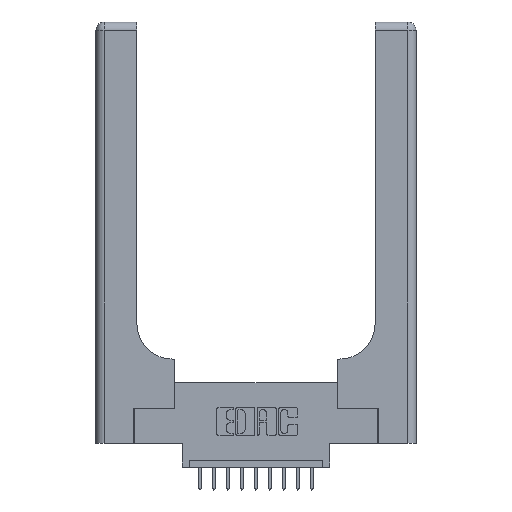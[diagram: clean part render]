
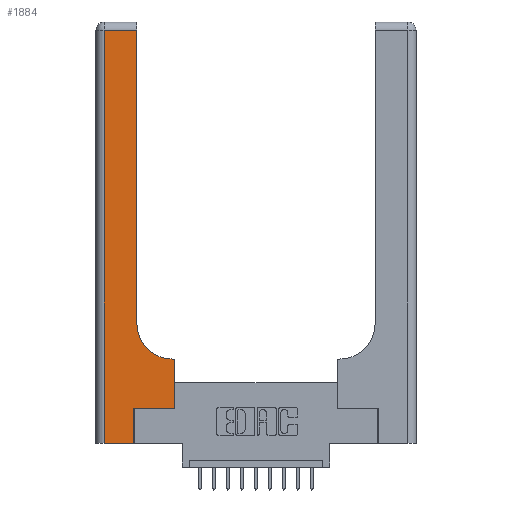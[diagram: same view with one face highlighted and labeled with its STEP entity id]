
A CAD part, top view. The second image highlights one B-rep face of the part: STEP entity #1884.
In plain terms, the highlighted planar face has unit normal (0, 0, 1).
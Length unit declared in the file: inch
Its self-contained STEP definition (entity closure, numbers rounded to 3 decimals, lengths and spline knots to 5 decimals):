
#224 = CARTESIAN_POINT ( 'NONE',  ( 0.2915, 0.6, 0.37 ) ) ;
#412 = VECTOR ( 'NONE', #5298, 39.37008 ) ;
#674 = FACE_OUTER_BOUND ( 'NONE', #16496, .T. ) ;
#1247 = EDGE_CURVE ( 'NONE', #13207, #6034, #7113, .T. ) ;
#1469 = VERTEX_POINT ( 'NONE', #1929 ) ;
#1557 = CARTESIAN_POINT ( 'NONE',  ( 0.06, 0., 0.37 ) ) ;
#1884 = ADVANCED_FACE ( 'NONE', ( #674 ), #8360, .F. ) ;
#1929 = CARTESIAN_POINT ( 'NONE',  ( 0.06, 2.94, 0.37 ) ) ;
#2017 = DIRECTION ( 'NONE',  ( -1., 0., 0. ) ) ;
#2790 = CARTESIAN_POINT ( 'NONE',  ( 0.2915, 3., 0.37 ) ) ;
#2985 = CARTESIAN_POINT ( 'NONE',  ( 0.5585, 0.25, 0.37 ) ) ;
#3104 = DIRECTION ( 'NONE',  ( 0., 1., 0. ) ) ;
#3157 = VECTOR ( 'NONE', #4562, 39.37008 ) ;
#3801 = EDGE_CURVE ( 'NONE', #5965, #1469, #4281, .T. ) ;
#3925 = CARTESIAN_POINT ( 'NONE',  ( 0.5415, 0.6, 0.37 ) ) ;
#3981 = DIRECTION ( 'NONE',  ( -1., 0., 0. ) ) ;
#4088 = DIRECTION ( 'NONE',  ( 0., 1., 0. ) ) ;
#4189 = CARTESIAN_POINT ( 'NONE',  ( 0.5415, 0.85, 0.37 ) ) ;
#4281 = LINE ( 'NONE', #15075, #5456 ) ;
#4562 = DIRECTION ( 'NONE',  ( 0., 1., 0. ) ) ;
#4927 = ORIENTED_EDGE ( 'NONE', *, *, #10710, .T. ) ;
#5298 = DIRECTION ( 'NONE',  ( 1., 0., 0. ) ) ;
#5456 = VECTOR ( 'NONE', #7388, 39.37008 ) ;
#5472 = LINE ( 'NONE', #10953, #6262 ) ;
#5574 = VERTEX_POINT ( 'NONE', #3925 ) ;
#5611 = ORIENTED_EDGE ( 'NONE', *, *, #8566, .T. ) ;
#5673 = LINE ( 'NONE', #2790, #9838 ) ;
#5813 = DIRECTION ( 'NONE',  ( 0., 0., -1. ) ) ;
#5936 = DIRECTION ( 'NONE',  ( 0., -1., 0. ) ) ;
#5965 = VERTEX_POINT ( 'NONE', #11740 ) ;
#5984 = CARTESIAN_POINT ( 'NONE',  ( 0.269, 0., 0.37 ) ) ;
#6010 = CARTESIAN_POINT ( 'NONE',  ( 0.269, 0.25, 0.37 ) ) ;
#6034 = VERTEX_POINT ( 'NONE', #6010 ) ;
#6070 = LINE ( 'NONE', #2985, #13276 ) ;
#6248 = ORIENTED_EDGE ( 'NONE', *, *, #9788, .T. ) ;
#6262 = VECTOR ( 'NONE', #5936, 39.37008 ) ;
#6464 = VECTOR ( 'NONE', #3981, 39.37008 ) ;
#7108 = ORIENTED_EDGE ( 'NONE', *, *, #3801, .T. ) ;
#7113 = LINE ( 'NONE', #5984, #3157 ) ;
#7388 = DIRECTION ( 'NONE',  ( -1., 0., 0. ) ) ;
#8030 = LINE ( 'NONE', #14194, #412 ) ;
#8059 = ORIENTED_EDGE ( 'NONE', *, *, #14907, .T. ) ;
#8360 = PLANE ( 'NONE',  #12251 ) ;
#8391 = CARTESIAN_POINT ( 'NONE',  ( 0.5585, 0.25, 0.37 ) ) ;
#8566 = EDGE_CURVE ( 'NONE', #5574, #14475, #8682, .T. ) ;
#8589 = VERTEX_POINT ( 'NONE', #15667 ) ;
#8682 = CIRCLE ( 'NONE', #15657, 0.25 ) ;
#9118 = ORIENTED_EDGE ( 'NONE', *, *, #1247, .T. ) ;
#9221 = LINE ( 'NONE', #224, #6464 ) ;
#9788 = EDGE_CURVE ( 'NONE', #13257, #8589, #6070, .T. ) ;
#9838 = VECTOR ( 'NONE', #4088, 39.37008 ) ;
#9841 = EDGE_CURVE ( 'NONE', #6034, #13257, #10455, .T. ) ;
#9959 = EDGE_CURVE ( 'NONE', #1469, #11561, #5472, .T. ) ;
#10455 = LINE ( 'NONE', #14553, #11872 ) ;
#10648 = DIRECTION ( 'NONE',  ( 1., 0., 0. ) ) ;
#10710 = EDGE_CURVE ( 'NONE', #11561, #13207, #8030, .T. ) ;
#10880 = CARTESIAN_POINT ( 'NONE',  ( 0., 3., 0.37 ) ) ;
#10953 = CARTESIAN_POINT ( 'NONE',  ( 0.06, 3., 0.37 ) ) ;
#11561 = VERTEX_POINT ( 'NONE', #1557 ) ;
#11740 = CARTESIAN_POINT ( 'NONE',  ( 0.2915, 2.94, 0.37 ) ) ;
#11872 = VECTOR ( 'NONE', #10648, 39.37008 ) ;
#12251 = AXIS2_PLACEMENT_3D ( 'NONE', #10880, #5813, #2017 ) ;
#12821 = ORIENTED_EDGE ( 'NONE', *, *, #9841, .T. ) ;
#12918 = DIRECTION ( 'NONE',  ( 0., 0., -1. ) ) ;
#13207 = VERTEX_POINT ( 'NONE', #16111 ) ;
#13257 = VERTEX_POINT ( 'NONE', #8391 ) ;
#13276 = VECTOR ( 'NONE', #3104, 39.37008 ) ;
#13300 = CARTESIAN_POINT ( 'NONE',  ( 0.2915, 0.85, 0.37 ) ) ;
#14042 = ORIENTED_EDGE ( 'NONE', *, *, #14946, .T. ) ;
#14194 = CARTESIAN_POINT ( 'NONE',  ( 0., 0., 0.37 ) ) ;
#14469 = ORIENTED_EDGE ( 'NONE', *, *, #9959, .T. ) ;
#14475 = VERTEX_POINT ( 'NONE', #13300 ) ;
#14553 = CARTESIAN_POINT ( 'NONE',  ( 0.269, 0.25, 0.37 ) ) ;
#14907 = EDGE_CURVE ( 'NONE', #14475, #5965, #5673, .T. ) ;
#14946 = EDGE_CURVE ( 'NONE', #8589, #5574, #9221, .T. ) ;
#15075 = CARTESIAN_POINT ( 'NONE',  ( 0., 2.94, 0.37 ) ) ;
#15553 = DIRECTION ( 'NONE',  ( 1., 0., 0. ) ) ;
#15657 = AXIS2_PLACEMENT_3D ( 'NONE', #4189, #12918, #15553 ) ;
#15667 = CARTESIAN_POINT ( 'NONE',  ( 0.5585, 0.6, 0.37 ) ) ;
#16111 = CARTESIAN_POINT ( 'NONE',  ( 0.269, 0., 0.37 ) ) ;
#16496 = EDGE_LOOP ( 'NONE', ( #8059, #7108, #14469, #4927, #9118, #12821, #6248, #14042, #5611 ) ) ;
